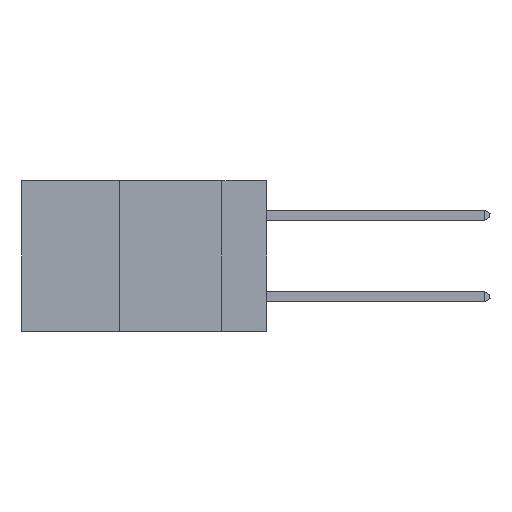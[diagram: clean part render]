
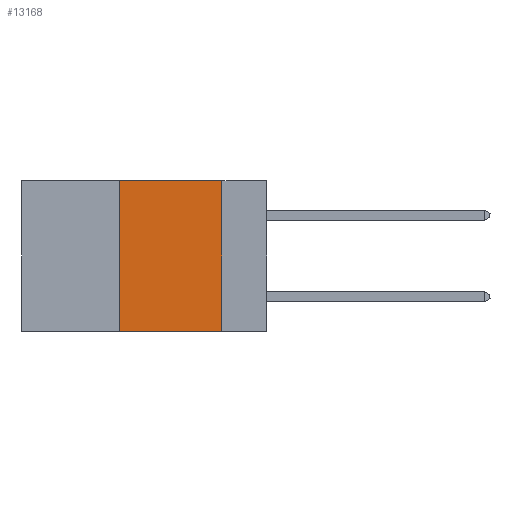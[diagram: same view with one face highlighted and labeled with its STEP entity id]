
A CAD part, left-side view. The second image highlights one B-rep face of the part: STEP entity #13168.
In plain terms, the highlighted planar face has unit normal (-1, 0, 0).
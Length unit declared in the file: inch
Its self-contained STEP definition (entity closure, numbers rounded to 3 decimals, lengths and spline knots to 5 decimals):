
#726 = PLANE ( 'NONE',  #14984 ) ;
#933 = LINE ( 'NONE', #8236, #28978 ) ;
#1350 = LINE ( 'NONE', #3834, #6731 ) ;
#1374 = VECTOR ( 'NONE', #3084, 39.37008 ) ;
#1577 = DIRECTION ( 'NONE',  ( 0., 0., -1. ) ) ;
#3084 = DIRECTION ( 'NONE',  ( 0., -1., 0. ) ) ;
#3834 = CARTESIAN_POINT ( 'NONE',  ( 0., 0.6, -0.37 ) ) ;
#3926 = DIRECTION ( 'NONE',  ( 0., -1., 0. ) ) ;
#4233 = LINE ( 'NONE', #7594, #1374 ) ;
#4700 = VERTEX_POINT ( 'NONE', #14700 ) ;
#6510 = EDGE_LOOP ( 'NONE', ( #29474, #13651, #18943, #12732 ) ) ;
#6731 = VECTOR ( 'NONE', #3926, 39.37008 ) ;
#6753 = DIRECTION ( 'NONE',  ( 0., 0., 1. ) ) ;
#6834 = VECTOR ( 'NONE', #6753, 39.37008 ) ;
#7594 = CARTESIAN_POINT ( 'NONE',  ( 0., 0.6, 0. ) ) ;
#7962 = LINE ( 'NONE', #20630, #6834 ) ;
#8236 = CARTESIAN_POINT ( 'NONE',  ( 0., 0.11, 0. ) ) ;
#9363 = EDGE_CURVE ( 'NONE', #4700, #9722, #1350, .T. ) ;
#9722 = VERTEX_POINT ( 'NONE', #20930 ) ;
#10755 = EDGE_CURVE ( 'NONE', #19146, #9722, #933, .T. ) ;
#12732 = ORIENTED_EDGE ( 'NONE', *, *, #9363, .T. ) ;
#13168 = ADVANCED_FACE ( 'NONE', ( #26351 ), #726, .F. ) ;
#13651 = ORIENTED_EDGE ( 'NONE', *, *, #23059, .F. ) ;
#14700 = CARTESIAN_POINT ( 'NONE',  ( 0., 0.36, -0.37 ) ) ;
#14984 = AXIS2_PLACEMENT_3D ( 'NONE', #16528, #18816, #21127 ) ;
#16528 = CARTESIAN_POINT ( 'NONE',  ( 0., 0.6, 0. ) ) ;
#18171 = VERTEX_POINT ( 'NONE', #28946 ) ;
#18816 = DIRECTION ( 'NONE',  ( 1., 0., 0. ) ) ;
#18943 = ORIENTED_EDGE ( 'NONE', *, *, #21671, .F. ) ;
#19146 = VERTEX_POINT ( 'NONE', #25332 ) ;
#20630 = CARTESIAN_POINT ( 'NONE',  ( 0., 0.36, 0. ) ) ;
#20930 = CARTESIAN_POINT ( 'NONE',  ( 0., 0.11, -0.37 ) ) ;
#21127 = DIRECTION ( 'NONE',  ( 0., 0., -1. ) ) ;
#21671 = EDGE_CURVE ( 'NONE', #4700, #18171, #7962, .T. ) ;
#23059 = EDGE_CURVE ( 'NONE', #18171, #19146, #4233, .T. ) ;
#25332 = CARTESIAN_POINT ( 'NONE',  ( 0., 0.11, 0. ) ) ;
#26351 = FACE_OUTER_BOUND ( 'NONE', #6510, .T. ) ;
#28946 = CARTESIAN_POINT ( 'NONE',  ( 0., 0.36, 0. ) ) ;
#28978 = VECTOR ( 'NONE', #1577, 39.37008 ) ;
#29474 = ORIENTED_EDGE ( 'NONE', *, *, #10755, .F. ) ;
